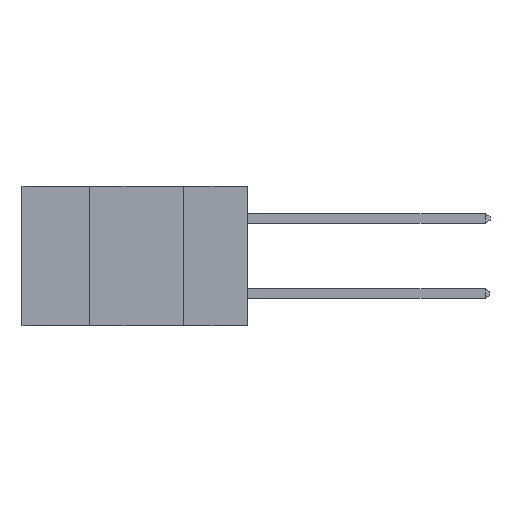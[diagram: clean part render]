
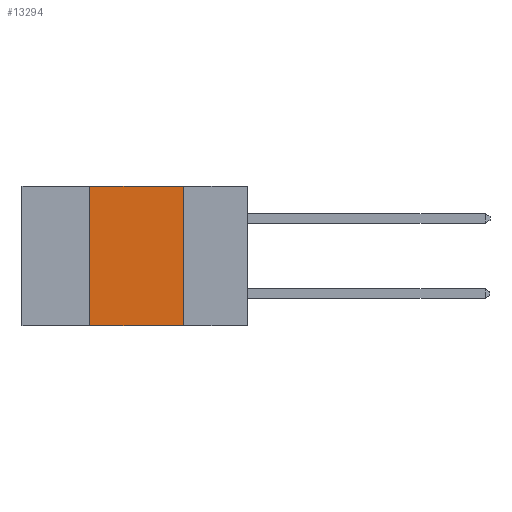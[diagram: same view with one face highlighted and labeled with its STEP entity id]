
A CAD part, left-side view. The second image highlights one B-rep face of the part: STEP entity #13294.
In plain terms, the highlighted planar face has unit normal (-1, 0, 0).
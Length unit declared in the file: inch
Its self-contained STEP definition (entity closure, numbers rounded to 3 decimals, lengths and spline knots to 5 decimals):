
#264 = LINE ( 'NONE', #711, #8573 ) ;
#711 = CARTESIAN_POINT ( 'NONE',  ( 0., 0.42, 0. ) ) ;
#1691 = DIRECTION ( 'NONE',  ( 0., -1., 0. ) ) ;
#1729 = DIRECTION ( 'NONE',  ( 0., 0., 1. ) ) ;
#1739 = DIRECTION ( 'NONE',  ( 1., 0., 0. ) ) ;
#1844 = CARTESIAN_POINT ( 'NONE',  ( 0., 0.17, -0.37 ) ) ;
#1848 = CARTESIAN_POINT ( 'NONE',  ( 0., 0.6, -0.37 ) ) ;
#2317 = ORIENTED_EDGE ( 'NONE', *, *, #12152, .F. ) ;
#3633 = CARTESIAN_POINT ( 'NONE',  ( 0., 0.17, 0. ) ) ;
#4423 = LINE ( 'NONE', #3633, #9612 ) ;
#4900 = CARTESIAN_POINT ( 'NONE',  ( 0., 0.6, 0. ) ) ;
#5056 = DIRECTION ( 'NONE',  ( 0., -1., 0. ) ) ;
#5209 = CARTESIAN_POINT ( 'NONE',  ( 0., 0.17, 0. ) ) ;
#7248 = EDGE_CURVE ( 'NONE', #9169, #11597, #8630, .T. ) ;
#7294 = VERTEX_POINT ( 'NONE', #13831 ) ;
#7351 = VERTEX_POINT ( 'NONE', #5209 ) ;
#7463 = CARTESIAN_POINT ( 'NONE',  ( 0., 0.42, -0.37 ) ) ;
#8274 = PLANE ( 'NONE',  #9166 ) ;
#8297 = VECTOR ( 'NONE', #5056, 39.37008 ) ;
#8573 = VECTOR ( 'NONE', #1729, 39.37008 ) ;
#8630 = LINE ( 'NONE', #1848, #8297 ) ;
#8890 = EDGE_CURVE ( 'NONE', #7351, #11597, #4423, .T. ) ;
#9166 = AXIS2_PLACEMENT_3D ( 'NONE', #13629, #1739, #9368 ) ;
#9169 = VERTEX_POINT ( 'NONE', #7463 ) ;
#9368 = DIRECTION ( 'NONE',  ( 0., 0., -1. ) ) ;
#9612 = VECTOR ( 'NONE', #12399, 39.37008 ) ;
#10009 = ORIENTED_EDGE ( 'NONE', *, *, #8890, .F. ) ;
#11139 = VECTOR ( 'NONE', #1691, 39.37008 ) ;
#11597 = VERTEX_POINT ( 'NONE', #1844 ) ;
#11671 = ORIENTED_EDGE ( 'NONE', *, *, #12153, .F. ) ;
#11694 = ORIENTED_EDGE ( 'NONE', *, *, #7248, .T. ) ;
#12152 = EDGE_CURVE ( 'NONE', #7294, #7351, #13956, .T. ) ;
#12153 = EDGE_CURVE ( 'NONE', #9169, #7294, #264, .T. ) ;
#12399 = DIRECTION ( 'NONE',  ( 0., 0., -1. ) ) ;
#12641 = EDGE_LOOP ( 'NONE', ( #10009, #2317, #11671, #11694 ) ) ;
#13294 = ADVANCED_FACE ( 'NONE', ( #13607 ), #8274, .F. ) ;
#13607 = FACE_OUTER_BOUND ( 'NONE', #12641, .T. ) ;
#13629 = CARTESIAN_POINT ( 'NONE',  ( 0., 0.6, 0. ) ) ;
#13831 = CARTESIAN_POINT ( 'NONE',  ( 0., 0.42, 0. ) ) ;
#13956 = LINE ( 'NONE', #4900, #11139 ) ;
